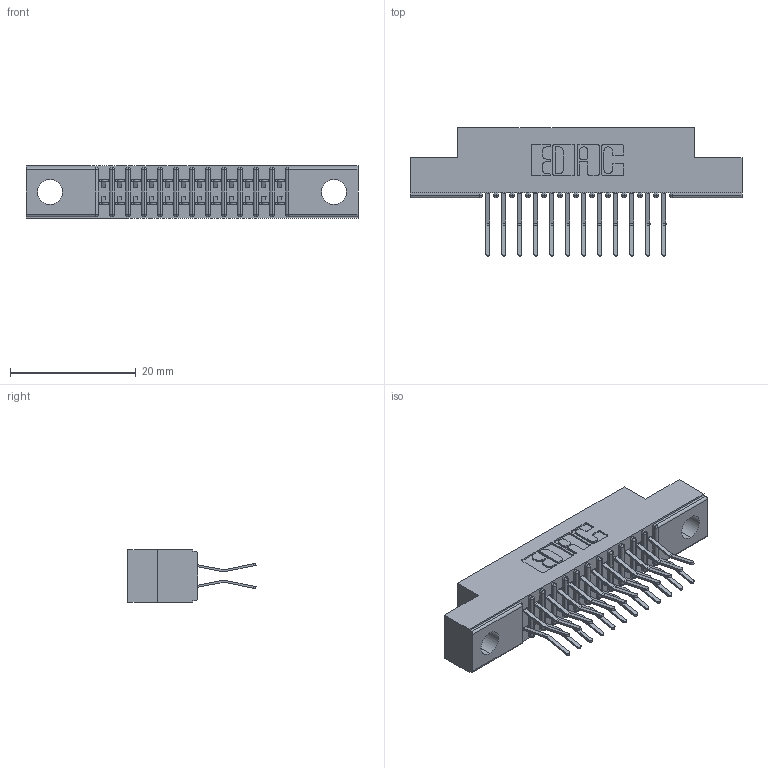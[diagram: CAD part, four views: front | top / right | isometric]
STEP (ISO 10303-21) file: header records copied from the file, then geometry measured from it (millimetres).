
FILE_DESCRIPTION (( 'STEP AP203' ), '1' );
FILE_NAME ('391-024-560-204.STEP', '2018-08-08T20:01:55', ( '' ), ( '' ), 'SwSTEP 2.0', 'SolidWorks 2016', '' );
FILE_SCHEMA (( 'CONFIG_CONTROL_DESIGN' ));
Length unit declared in the file: inch
Products named in the file (3): 341 Part_.156 (3.96) Dia Mounting Holes; 341-292-001_341-292-160; 391-024-560-204
Assembly tree (25 placements, depth 2):
  391-024-560-204
    341 Part_.156 (3.96) Dia Mounting Holes
    341-292-001_341-292-160  x24
Bounding box: 52.7 x 20.37 x 8.38 mm (x, y, z)
Volume: 2945.7 mm3; surface area: 5608.9 mm2
Topology: 25 solids, 25 shells, 1810 faces, 5236 edges, 3398 vertices
Faces by surface type: plane 1042, cylinder 720, sphere 26, torus 22
Entity records: 19077 total; most frequent: CARTESIAN_POINT 3178, ORIENTED_EDGE 3152, DIRECTION 3102, EDGE_CURVE 1576, VECTOR 1242, LINE 1242, VERTEX_POINT 1006, AXIS2_PLACEMENT_3D 930
